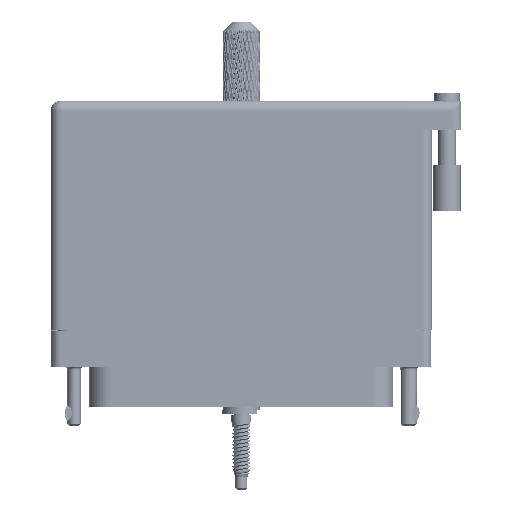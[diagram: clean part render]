
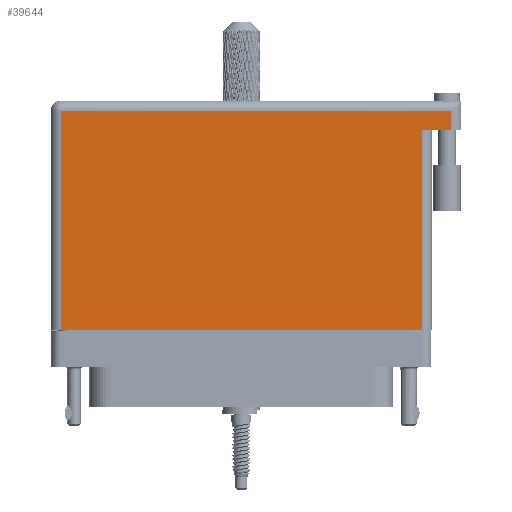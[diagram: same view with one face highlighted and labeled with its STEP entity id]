
A CAD part, front view. The second image highlights one B-rep face of the part: STEP entity #39644.
In plain terms, the highlighted face is planar.
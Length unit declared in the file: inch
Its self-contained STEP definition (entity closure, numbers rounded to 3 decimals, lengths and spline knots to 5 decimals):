
#622 = DIRECTION ( 'NONE',  ( -1., 0., 0. ) ) ;
#4020 = CARTESIAN_POINT ( 'NONE',  ( -1.23, 1.396, 0.4495 ) ) ;
#4289 = LINE ( 'NONE', #36875, #8864 ) ;
#5309 = CARTESIAN_POINT ( 'NONE',  ( 1.23, 1.269, 0.4495 ) ) ;
#8864 = VECTOR ( 'NONE', #35641, 39.37008 ) ;
#10363 = CARTESIAN_POINT ( 'NONE',  ( 1.23, -0.1, 0.4495 ) ) ;
#16521 = EDGE_CURVE ( 'NONE', #99582, #114825, #81048, .T. ) ;
#18751 = VERTEX_POINT ( 'NONE', #93019 ) ;
#24033 = EDGE_CURVE ( 'NONE', #57069, #114825, #4289, .T. ) ;
#24697 = ORIENTED_EDGE ( 'NONE', *, *, #24033, .F. ) ;
#29400 = CARTESIAN_POINT ( 'NONE',  ( -1.3, 1.396, 0.4495 ) ) ;
#32770 = DIRECTION ( 'NONE',  ( 0., 1., 0. ) ) ;
#33569 = VECTOR ( 'NONE', #92867, 39.37008 ) ;
#34175 = CARTESIAN_POINT ( 'NONE',  ( 1.43, 1.269, 0.4495 ) ) ;
#35641 = DIRECTION ( 'NONE',  ( -1., 0., 0. ) ) ;
#36875 = CARTESIAN_POINT ( 'NONE',  ( 1.5, 1.269, 0.4495 ) ) ;
#39644 = ADVANCED_FACE ( 'NONE', ( #41485 ), #89360, .F. ) ;
#39837 = VECTOR ( 'NONE', #49429, 39.37008 ) ;
#41485 = FACE_OUTER_BOUND ( 'NONE', #97640, .T. ) ;
#42761 = VECTOR ( 'NONE', #49557, 39.37008 ) ;
#49223 = DIRECTION ( 'NONE',  ( 0., 0., -1. ) ) ;
#49429 = DIRECTION ( 'NONE',  ( -1., 0., 0. ) ) ;
#49557 = DIRECTION ( 'NONE',  ( 0., -1., 0. ) ) ;
#57069 = VERTEX_POINT ( 'NONE', #34175 ) ;
#61764 = VERTEX_POINT ( 'NONE', #63360 ) ;
#63360 = CARTESIAN_POINT ( 'NONE',  ( -1.23, -0.1, 0.4495 ) ) ;
#64434 = ORIENTED_EDGE ( 'NONE', *, *, #16521, .T. ) ;
#64728 = LINE ( 'NONE', #100707, #110513 ) ;
#66000 = CARTESIAN_POINT ( 'NONE',  ( 1.23, 1.269, 0.4495 ) ) ;
#68355 = ORIENTED_EDGE ( 'NONE', *, *, #117838, .T. ) ;
#72064 = VERTEX_POINT ( 'NONE', #4020 ) ;
#72505 = EDGE_CURVE ( 'NONE', #72064, #61764, #102364, .T. ) ;
#74069 = ORIENTED_EDGE ( 'NONE', *, *, #120729, .T. ) ;
#75804 = VECTOR ( 'NONE', #89624, 39.37008 ) ;
#77927 = CARTESIAN_POINT ( 'NONE',  ( -1.3, 1.466, 0.4495 ) ) ;
#81048 = LINE ( 'NONE', #5309, #33569 ) ;
#85956 = ORIENTED_EDGE ( 'NONE', *, *, #98862, .T. ) ;
#89360 = PLANE ( 'NONE',  #116951 ) ;
#89624 = DIRECTION ( 'NONE',  ( 1., 0., 0. ) ) ;
#92867 = DIRECTION ( 'NONE',  ( 0., 1., 0. ) ) ;
#93019 = CARTESIAN_POINT ( 'NONE',  ( 1.43, 1.396, 0.4495 ) ) ;
#93342 = LINE ( 'NONE', #29400, #39837 ) ;
#97640 = EDGE_LOOP ( 'NONE', ( #68355, #64434, #24697, #74069, #85956, #106747 ) ) ;
#98733 = CARTESIAN_POINT ( 'NONE',  ( -1.23, -0.1, 0.4495 ) ) ;
#98862 = EDGE_CURVE ( 'NONE', #18751, #72064, #93342, .T. ) ;
#99582 = VERTEX_POINT ( 'NONE', #10363 ) ;
#100707 = CARTESIAN_POINT ( 'NONE',  ( 1.43, 1.466, 0.4495 ) ) ;
#102364 = LINE ( 'NONE', #98733, #42761 ) ;
#106747 = ORIENTED_EDGE ( 'NONE', *, *, #72505, .T. ) ;
#110513 = VECTOR ( 'NONE', #32770, 39.37008 ) ;
#114825 = VERTEX_POINT ( 'NONE', #66000 ) ;
#116951 = AXIS2_PLACEMENT_3D ( 'NONE', #77927, #49223, #622 ) ;
#117838 = EDGE_CURVE ( 'NONE', #61764, #99582, #118571, .T. ) ;
#118571 = LINE ( 'NONE', #119514, #75804 ) ;
#119514 = CARTESIAN_POINT ( 'NONE',  ( -1.3, -0.1, 0.4495 ) ) ;
#120729 = EDGE_CURVE ( 'NONE', #57069, #18751, #64728, .T. ) ;
